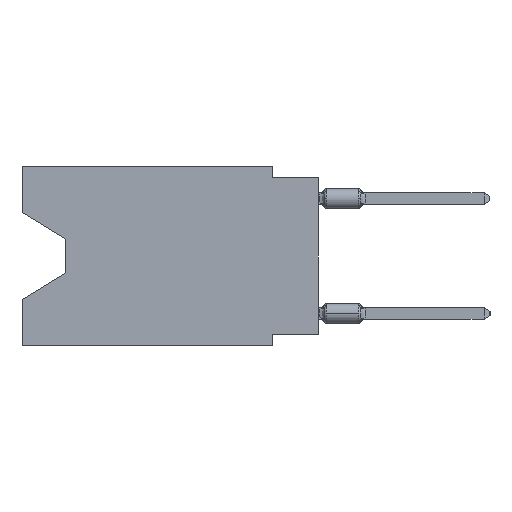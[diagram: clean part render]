
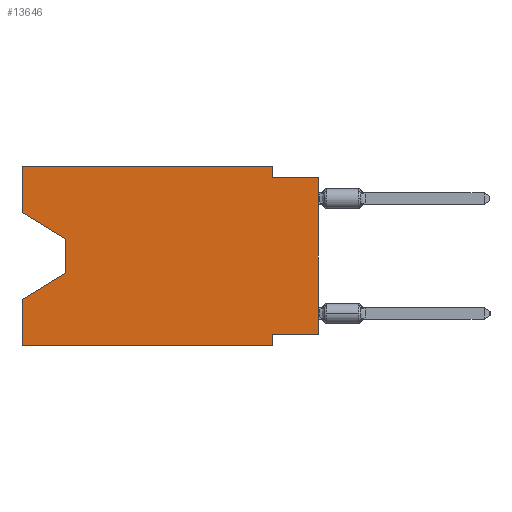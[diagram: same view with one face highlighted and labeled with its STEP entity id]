
A CAD part, left-side view. The second image highlights one B-rep face of the part: STEP entity #13646.
In plain terms, the highlighted planar face has unit normal (-1, 0, 0).
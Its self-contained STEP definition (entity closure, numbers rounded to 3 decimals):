
#64 = VERTEX_POINT ( 'NONE', #15860 ) ;
#789 = ORIENTED_EDGE ( 'NONE', *, *, #14100, .F. ) ;
#806 = LINE ( 'NONE', #36754, #57190 ) ;
#889 = DIRECTION ( 'NONE',  ( 0., 0., -1. ) ) ;
#978 = LINE ( 'NONE', #50401, #19553 ) ;
#1088 = CARTESIAN_POINT ( 'NONE',  ( 0., 2.54, 0. ) ) ;
#1249 = EDGE_CURVE ( 'NONE', #37233, #1708, #1646, .T. ) ;
#1646 = LINE ( 'NONE', #50506, #56308 ) ;
#1708 = VERTEX_POINT ( 'NONE', #7893 ) ;
#2566 = DIRECTION ( 'NONE',  ( 1., 0., 0. ) ) ;
#2687 = ORIENTED_EDGE ( 'NONE', *, *, #36842, .F. ) ;
#3730 = VERTEX_POINT ( 'NONE', #11363 ) ;
#5100 = DIRECTION ( 'NONE',  ( 0., -0.855, -0.519 ) ) ;
#5269 = EDGE_CURVE ( 'NONE', #3730, #33985, #54367, .T. ) ;
#5696 = CARTESIAN_POINT ( 'NONE',  ( 0., 16.383, -7.36 ) ) ;
#5836 = CARTESIAN_POINT ( 'NONE',  ( 0., 13.97, -4.013 ) ) ;
#6379 = ORIENTED_EDGE ( 'NONE', *, *, #57703, .T. ) ;
#6459 = DIRECTION ( 'NONE',  ( 0., -1., 0. ) ) ;
#6889 = DIRECTION ( 'NONE',  ( 0., -1., 0. ) ) ;
#7700 = DIRECTION ( 'NONE',  ( 0., 0., 1. ) ) ;
#7818 = DIRECTION ( 'NONE',  ( 0., 0., -1. ) ) ;
#7893 = CARTESIAN_POINT ( 'NONE',  ( 0., 0., -0.635 ) ) ;
#9258 = ORIENTED_EDGE ( 'NONE', *, *, #18976, .T. ) ;
#9484 = VERTEX_POINT ( 'NONE', #22021 ) ;
#9605 = ORIENTED_EDGE ( 'NONE', *, *, #5269, .F. ) ;
#9655 = LINE ( 'NONE', #5836, #40406 ) ;
#10580 = EDGE_CURVE ( 'NONE', #9484, #36864, #40685, .T. ) ;
#11363 = CARTESIAN_POINT ( 'NONE',  ( 0., 0., -9.271 ) ) ;
#13593 = DIRECTION ( 'NONE',  ( 0., 0., 1. ) ) ;
#13646 = ADVANCED_FACE ( 'NONE', ( #24748 ), #20653, .F. ) ;
#13844 = VECTOR ( 'NONE', #6459, 1000. ) ;
#14100 = EDGE_CURVE ( 'NONE', #20071, #42709, #55322, .T. ) ;
#14655 = ORIENTED_EDGE ( 'NONE', *, *, #24122, .T. ) ;
#15860 = CARTESIAN_POINT ( 'NONE',  ( 0., 13.97, -4.013 ) ) ;
#16130 = EDGE_LOOP ( 'NONE', ( #32075, #6379, #28721, #2687, #14655, #46575, #9605, #9258, #19513, #24823, #789, #38309 ) ) ;
#18615 = CARTESIAN_POINT ( 'NONE',  ( 0., 2.54, -9.271 ) ) ;
#18976 = EDGE_CURVE ( 'NONE', #3730, #1708, #29612, .T. ) ;
#19281 = CARTESIAN_POINT ( 'NONE',  ( 0., 2.54, -9.906 ) ) ;
#19513 = ORIENTED_EDGE ( 'NONE', *, *, #1249, .F. ) ;
#19553 = VECTOR ( 'NONE', #45421, 1000. ) ;
#20012 = CARTESIAN_POINT ( 'NONE',  ( 0., 16.383, -9.906 ) ) ;
#20071 = VERTEX_POINT ( 'NONE', #40239 ) ;
#20327 = VECTOR ( 'NONE', #7700, 1000. ) ;
#20599 = EDGE_CURVE ( 'NONE', #46358, #20071, #978, .T. ) ;
#20653 = PLANE ( 'NONE',  #25133 ) ;
#21913 = EDGE_CURVE ( 'NONE', #46358, #64, #54261, .T. ) ;
#22021 = CARTESIAN_POINT ( 'NONE',  ( 0., 13.97, -5.893 ) ) ;
#22700 = DIRECTION ( 'NONE',  ( 0., 0., -1. ) ) ;
#22740 = VECTOR ( 'NONE', #13593, 1000. ) ;
#23735 = CARTESIAN_POINT ( 'NONE',  ( 0., 2.54, 0. ) ) ;
#24122 = EDGE_CURVE ( 'NONE', #31271, #29391, #52238, .T. ) ;
#24748 = FACE_OUTER_BOUND ( 'NONE', #16130, .T. ) ;
#24823 = ORIENTED_EDGE ( 'NONE', *, *, #49653, .F. ) ;
#25133 = AXIS2_PLACEMENT_3D ( 'NONE', #33858, #2566, #7818 ) ;
#25808 = VECTOR ( 'NONE', #49983, 1000. ) ;
#28659 = CARTESIAN_POINT ( 'NONE',  ( 0., 16.383, 0. ) ) ;
#28721 = ORIENTED_EDGE ( 'NONE', *, *, #10580, .T. ) ;
#29391 = VERTEX_POINT ( 'NONE', #19281 ) ;
#29612 = LINE ( 'NONE', #47186, #20327 ) ;
#30445 = CARTESIAN_POINT ( 'NONE',  ( 0., 13.97, -5.893 ) ) ;
#31271 = VERTEX_POINT ( 'NONE', #20012 ) ;
#31372 = CARTESIAN_POINT ( 'NONE',  ( 0., 2.54, -0.635 ) ) ;
#31924 = CARTESIAN_POINT ( 'NONE',  ( 0., 16.383, -2.546 ) ) ;
#32075 = ORIENTED_EDGE ( 'NONE', *, *, #21913, .T. ) ;
#33008 = EDGE_CURVE ( 'NONE', #33985, #29391, #806, .T. ) ;
#33050 = DIRECTION ( 'NONE',  ( 0., 0.855, -0.519 ) ) ;
#33858 = CARTESIAN_POINT ( 'NONE',  ( 0., 16.383, 0. ) ) ;
#33985 = VERTEX_POINT ( 'NONE', #18615 ) ;
#35826 = CARTESIAN_POINT ( 'NONE',  ( 0., 16.383, 0. ) ) ;
#36748 = LINE ( 'NONE', #1088, #40939 ) ;
#36754 = CARTESIAN_POINT ( 'NONE',  ( 0., 2.54, -9.906 ) ) ;
#36842 = EDGE_CURVE ( 'NONE', #31271, #36864, #49021, .T. ) ;
#36864 = VERTEX_POINT ( 'NONE', #5696 ) ;
#37233 = VERTEX_POINT ( 'NONE', #31372 ) ;
#38091 = DIRECTION ( 'NONE',  ( 0., 0., -1. ) ) ;
#38180 = VECTOR ( 'NONE', #6889, 1000. ) ;
#38309 = ORIENTED_EDGE ( 'NONE', *, *, #20599, .F. ) ;
#39269 = VECTOR ( 'NONE', #33050, 1000. ) ;
#40239 = CARTESIAN_POINT ( 'NONE',  ( 0., 16.383, 0. ) ) ;
#40406 = VECTOR ( 'NONE', #889, 1000. ) ;
#40685 = LINE ( 'NONE', #30445, #39269 ) ;
#40939 = VECTOR ( 'NONE', #22700, 1000. ) ;
#41423 = DIRECTION ( 'NONE',  ( 0., -1., 0. ) ) ;
#42423 = CARTESIAN_POINT ( 'NONE',  ( 0., 16.383, -2.546 ) ) ;
#42709 = VERTEX_POINT ( 'NONE', #23735 ) ;
#43170 = CARTESIAN_POINT ( 'NONE',  ( 0., 16.383, -9.906 ) ) ;
#45421 = DIRECTION ( 'NONE',  ( 0., 0., 1. ) ) ;
#46358 = VERTEX_POINT ( 'NONE', #31924 ) ;
#46575 = ORIENTED_EDGE ( 'NONE', *, *, #33008, .F. ) ;
#47186 = CARTESIAN_POINT ( 'NONE',  ( 0., 0., 0. ) ) ;
#47425 = VECTOR ( 'NONE', #5100, 1000. ) ;
#49021 = LINE ( 'NONE', #35826, #22740 ) ;
#49653 = EDGE_CURVE ( 'NONE', #42709, #37233, #36748, .T. ) ;
#49983 = DIRECTION ( 'NONE',  ( 0., 1., 0. ) ) ;
#50401 = CARTESIAN_POINT ( 'NONE',  ( 0., 16.383, 0. ) ) ;
#50506 = CARTESIAN_POINT ( 'NONE',  ( 0., 0., -0.635 ) ) ;
#52238 = LINE ( 'NONE', #43170, #38180 ) ;
#54261 = LINE ( 'NONE', #42423, #47425 ) ;
#54367 = LINE ( 'NONE', #54939, #25808 ) ;
#54939 = CARTESIAN_POINT ( 'NONE',  ( 0., 0., -9.271 ) ) ;
#55322 = LINE ( 'NONE', #28659, #13844 ) ;
#56308 = VECTOR ( 'NONE', #41423, 1000. ) ;
#57190 = VECTOR ( 'NONE', #38091, 1000. ) ;
#57703 = EDGE_CURVE ( 'NONE', #64, #9484, #9655, .T. ) ;
